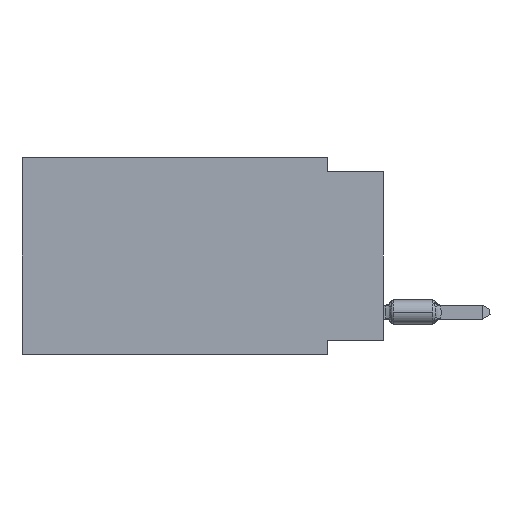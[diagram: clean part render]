
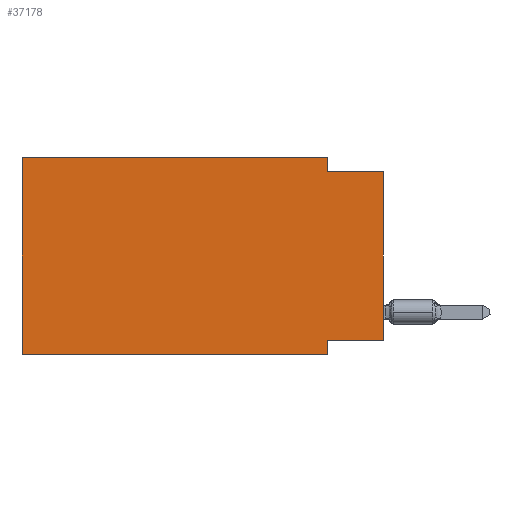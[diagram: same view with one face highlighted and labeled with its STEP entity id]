
A CAD part, left-side view. The second image highlights one B-rep face of the part: STEP entity #37178.
In plain terms, the highlighted planar face has unit normal (-1, 0, 0).
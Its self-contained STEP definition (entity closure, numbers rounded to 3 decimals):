
#2154 = DIRECTION ( 'NONE',  ( 0., 0., -1. ) ) ;
#2379 = VECTOR ( 'NONE', #24293, 1000. ) ;
#2477 = EDGE_CURVE ( 'NONE', #35282, #10858, #56724, .T. ) ;
#3005 = DIRECTION ( 'NONE',  ( 0., 0., 1. ) ) ;
#4137 = ORIENTED_EDGE ( 'NONE', *, *, #2477, .F. ) ;
#4176 = EDGE_CURVE ( 'NONE', #10858, #52019, #12236, .T. ) ;
#4832 = DIRECTION ( 'NONE',  ( 0., 0., -1. ) ) ;
#5413 = VECTOR ( 'NONE', #26839, 1000. ) ;
#5840 = CARTESIAN_POINT ( 'NONE',  ( 0., 2.54, 0. ) ) ;
#6065 = EDGE_CURVE ( 'NONE', #51595, #52384, #47877, .T. ) ;
#6792 = CARTESIAN_POINT ( 'NONE',  ( 0., 0., 0. ) ) ;
#6953 = VECTOR ( 'NONE', #52507, 1000. ) ;
#8130 = CARTESIAN_POINT ( 'NONE',  ( 0., 2.54, -8.89 ) ) ;
#10542 = LINE ( 'NONE', #42833, #12020 ) ;
#10858 = VERTEX_POINT ( 'NONE', #45507 ) ;
#12020 = VECTOR ( 'NONE', #19373, 1000. ) ;
#12236 = LINE ( 'NONE', #18011, #5413 ) ;
#15276 = DIRECTION ( 'NONE',  ( 0., 0., -1. ) ) ;
#15862 = CARTESIAN_POINT ( 'NONE',  ( 0., 2.54, -8.89 ) ) ;
#17035 = LINE ( 'NONE', #45065, #57315 ) ;
#17263 = VECTOR ( 'NONE', #15276, 1000. ) ;
#17742 = EDGE_CURVE ( 'NONE', #27325, #52019, #57658, .T. ) ;
#18011 = CARTESIAN_POINT ( 'NONE',  ( 0., 0., -0.635 ) ) ;
#19166 = LINE ( 'NONE', #56335, #2379 ) ;
#19233 = CARTESIAN_POINT ( 'NONE',  ( 0., 2.54, 0. ) ) ;
#19373 = DIRECTION ( 'NONE',  ( 0., -1., 0. ) ) ;
#19605 = EDGE_CURVE ( 'NONE', #34622, #35282, #10542, .T. ) ;
#19762 = AXIS2_PLACEMENT_3D ( 'NONE', #50557, #22811, #4832 ) ;
#20938 = CARTESIAN_POINT ( 'NONE',  ( 0., 16.383, 0. ) ) ;
#22811 = DIRECTION ( 'NONE',  ( 1., 0., 0. ) ) ;
#24293 = DIRECTION ( 'NONE',  ( 0., -1., 0. ) ) ;
#24873 = ORIENTED_EDGE ( 'NONE', *, *, #43599, .F. ) ;
#26407 = VERTEX_POINT ( 'NONE', #44049 ) ;
#26839 = DIRECTION ( 'NONE',  ( 0., -1., 0. ) ) ;
#27325 = VERTEX_POINT ( 'NONE', #48619 ) ;
#28632 = VECTOR ( 'NONE', #2154, 1000. ) ;
#29304 = ORIENTED_EDGE ( 'NONE', *, *, #19605, .F. ) ;
#32999 = CARTESIAN_POINT ( 'NONE',  ( 0., 2.54, -8.255 ) ) ;
#34622 = VERTEX_POINT ( 'NONE', #20938 ) ;
#35282 = VERTEX_POINT ( 'NONE', #19233 ) ;
#35379 = CARTESIAN_POINT ( 'NONE',  ( 0., 0., -0.635 ) ) ;
#37178 = ADVANCED_FACE ( 'NONE', ( #41731 ), #51171, .F. ) ;
#41731 = FACE_OUTER_BOUND ( 'NONE', #50574, .T. ) ;
#42833 = CARTESIAN_POINT ( 'NONE',  ( 0., 16.383, 0. ) ) ;
#43599 = EDGE_CURVE ( 'NONE', #27325, #51595, #45546, .T. ) ;
#43973 = ORIENTED_EDGE ( 'NONE', *, *, #54702, .F. ) ;
#44049 = CARTESIAN_POINT ( 'NONE',  ( 0., 16.383, -8.89 ) ) ;
#45065 = CARTESIAN_POINT ( 'NONE',  ( 0., 16.383, 0. ) ) ;
#45507 = CARTESIAN_POINT ( 'NONE',  ( 0., 2.54, -0.635 ) ) ;
#45546 = LINE ( 'NONE', #54366, #53802 ) ;
#45592 = ORIENTED_EDGE ( 'NONE', *, *, #17742, .T. ) ;
#47877 = LINE ( 'NONE', #15862, #17263 ) ;
#48619 = CARTESIAN_POINT ( 'NONE',  ( 0., 0., -8.255 ) ) ;
#50557 = CARTESIAN_POINT ( 'NONE',  ( 0., 16.383, 0. ) ) ;
#50574 = EDGE_LOOP ( 'NONE', ( #45592, #59093, #4137, #29304, #43973, #60144, #52068, #24873 ) ) ;
#51171 = PLANE ( 'NONE',  #19762 ) ;
#51595 = VERTEX_POINT ( 'NONE', #32999 ) ;
#52019 = VERTEX_POINT ( 'NONE', #35379 ) ;
#52068 = ORIENTED_EDGE ( 'NONE', *, *, #6065, .F. ) ;
#52384 = VERTEX_POINT ( 'NONE', #8130 ) ;
#52507 = DIRECTION ( 'NONE',  ( 0., 0., 1. ) ) ;
#53802 = VECTOR ( 'NONE', #54972, 1000. ) ;
#54366 = CARTESIAN_POINT ( 'NONE',  ( 0., 0., -8.255 ) ) ;
#54702 = EDGE_CURVE ( 'NONE', #26407, #34622, #17035, .T. ) ;
#54972 = DIRECTION ( 'NONE',  ( 0., 1., 0. ) ) ;
#56291 = EDGE_CURVE ( 'NONE', #26407, #52384, #19166, .T. ) ;
#56335 = CARTESIAN_POINT ( 'NONE',  ( 0., 16.383, -8.89 ) ) ;
#56724 = LINE ( 'NONE', #5840, #28632 ) ;
#57315 = VECTOR ( 'NONE', #3005, 1000. ) ;
#57658 = LINE ( 'NONE', #6792, #6953 ) ;
#59093 = ORIENTED_EDGE ( 'NONE', *, *, #4176, .F. ) ;
#60144 = ORIENTED_EDGE ( 'NONE', *, *, #56291, .T. ) ;
